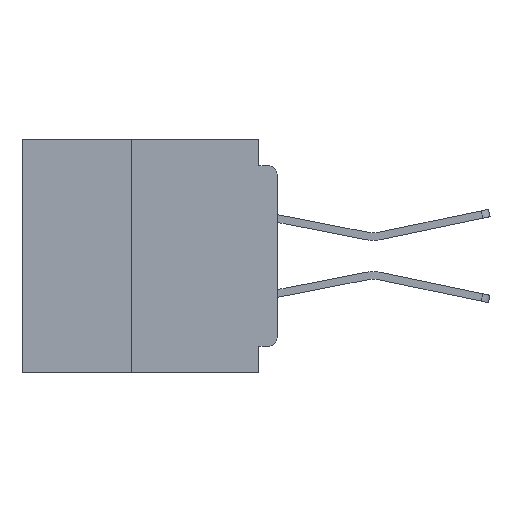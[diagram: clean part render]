
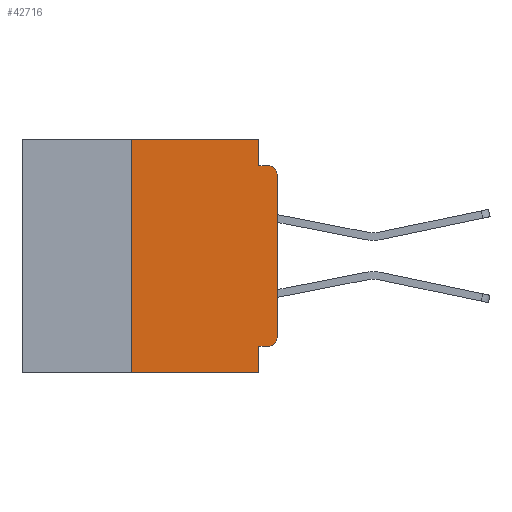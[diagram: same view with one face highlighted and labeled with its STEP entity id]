
A CAD part, left-side view. The second image highlights one B-rep face of the part: STEP entity #42716.
In plain terms, the highlighted planar face has unit normal (-1, 0, 0).
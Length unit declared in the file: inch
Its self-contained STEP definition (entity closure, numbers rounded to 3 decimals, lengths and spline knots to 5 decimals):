
#60 = CARTESIAN_POINT ( 'NONE',  ( 0., 0.015, -0.045 ) ) ;
#871 = ORIENTED_EDGE ( 'NONE', *, *, #28045, .T. ) ;
#939 = CARTESIAN_POINT ( 'NONE',  ( 0., 0., -0.355 ) ) ;
#1099 = CARTESIAN_POINT ( 'NONE',  ( 0., 0.031, -0.355 ) ) ;
#1116 = EDGE_CURVE ( 'NONE', #34935, #12988, #36839, .T. ) ;
#1674 = DIRECTION ( 'NONE',  ( 0., 1., 0. ) ) ;
#2947 = DIRECTION ( 'NONE',  ( 0., 0., 1. ) ) ;
#3328 = VERTEX_POINT ( 'NONE', #26756 ) ;
#4204 = CARTESIAN_POINT ( 'NONE',  ( 0., 0.031, 0. ) ) ;
#4971 = EDGE_LOOP ( 'NONE', ( #45256, #871, #13522, #13815, #39506, #6756, #7369, #54863, #20001, #50332 ) ) ;
#5549 = AXIS2_PLACEMENT_3D ( 'NONE', #36552, #10445, #40880 ) ;
#6756 = ORIENTED_EDGE ( 'NONE', *, *, #45501, .F. ) ;
#7180 = CARTESIAN_POINT ( 'NONE',  ( 0., 0.25, -0.4 ) ) ;
#7369 = ORIENTED_EDGE ( 'NONE', *, *, #21340, .T. ) ;
#7827 = CARTESIAN_POINT ( 'NONE',  ( 0., 0.031, 0. ) ) ;
#8248 = VERTEX_POINT ( 'NONE', #51144 ) ;
#9080 = VECTOR ( 'NONE', #18719, 39.37008 ) ;
#10445 = DIRECTION ( 'NONE',  ( -1., 0., 0. ) ) ;
#11455 = LINE ( 'NONE', #29660, #33284 ) ;
#12564 = CIRCLE ( 'NONE', #5549, 0.015 ) ;
#12753 = EDGE_CURVE ( 'NONE', #20427, #3328, #43786, .T. ) ;
#12988 = VERTEX_POINT ( 'NONE', #1099 ) ;
#13173 = LINE ( 'NONE', #17476, #23426 ) ;
#13522 = ORIENTED_EDGE ( 'NONE', *, *, #47722, .F. ) ;
#13557 = DIRECTION ( 'NONE',  ( 0., -1., 0. ) ) ;
#13815 = ORIENTED_EDGE ( 'NONE', *, *, #34812, .F. ) ;
#17476 = CARTESIAN_POINT ( 'NONE',  ( 0., 0.437, -0.4 ) ) ;
#18516 = EDGE_CURVE ( 'NONE', #36464, #53913, #11455, .T. ) ;
#18719 = DIRECTION ( 'NONE',  ( 0., 0., 1. ) ) ;
#18910 = AXIS2_PLACEMENT_3D ( 'NONE', #22741, #31313, #31490 ) ;
#20001 = ORIENTED_EDGE ( 'NONE', *, *, #1116, .F. ) ;
#20389 = VECTOR ( 'NONE', #49012, 39.37008 ) ;
#20427 = VERTEX_POINT ( 'NONE', #54319 ) ;
#21340 = EDGE_CURVE ( 'NONE', #31365, #35934, #13173, .T. ) ;
#21766 = LINE ( 'NONE', #31767, #20389 ) ;
#22258 = EDGE_CURVE ( 'NONE', #12988, #35934, #21766, .T. ) ;
#22369 = CARTESIAN_POINT ( 'NONE',  ( 0., 0., -0.045 ) ) ;
#22741 = CARTESIAN_POINT ( 'NONE',  ( 0., 0.437, 0. ) ) ;
#23426 = VECTOR ( 'NONE', #39134, 39.37008 ) ;
#24637 = VECTOR ( 'NONE', #2947, 39.37008 ) ;
#25216 = DIRECTION ( 'NONE',  ( 0., 0., -1. ) ) ;
#25240 = VECTOR ( 'NONE', #1674, 39.37008 ) ;
#25669 = CARTESIAN_POINT ( 'NONE',  ( 0., 0.015, -0.06 ) ) ;
#26756 = CARTESIAN_POINT ( 'NONE',  ( 0., 0., -0.06 ) ) ;
#27096 = PLANE ( 'NONE',  #18910 ) ;
#28045 = EDGE_CURVE ( 'NONE', #3328, #29928, #29028, .T. ) ;
#28723 = CARTESIAN_POINT ( 'NONE',  ( 0., 0.031, -0.4 ) ) ;
#29028 = CIRCLE ( 'NONE', #44156, 0.015 ) ;
#29503 = EDGE_CURVE ( 'NONE', #34935, #20427, #12564, .T. ) ;
#29660 = CARTESIAN_POINT ( 'NONE',  ( 0., 0.437, 0. ) ) ;
#29928 = VERTEX_POINT ( 'NONE', #60 ) ;
#30041 = DIRECTION ( 'NONE',  ( 0., 0., -1. ) ) ;
#31313 = DIRECTION ( 'NONE',  ( 1., 0., 0. ) ) ;
#31365 = VERTEX_POINT ( 'NONE', #36848 ) ;
#31490 = DIRECTION ( 'NONE',  ( 0., 0., -1. ) ) ;
#31625 = CARTESIAN_POINT ( 'NONE',  ( 0., 0., 0. ) ) ;
#31767 = CARTESIAN_POINT ( 'NONE',  ( 0., 0.031, -0.4 ) ) ;
#33284 = VECTOR ( 'NONE', #34023, 39.37008 ) ;
#34023 = DIRECTION ( 'NONE',  ( 0., -1., 0. ) ) ;
#34812 = EDGE_CURVE ( 'NONE', #53913, #8248, #37927, .T. ) ;
#34935 = VERTEX_POINT ( 'NONE', #52120 ) ;
#35934 = VERTEX_POINT ( 'NONE', #28723 ) ;
#36226 = LINE ( 'NONE', #7180, #24637 ) ;
#36368 = CARTESIAN_POINT ( 'NONE',  ( 0., 0.25, 0. ) ) ;
#36464 = VERTEX_POINT ( 'NONE', #36368 ) ;
#36552 = CARTESIAN_POINT ( 'NONE',  ( 0., 0.015, -0.34 ) ) ;
#36554 = VECTOR ( 'NONE', #25216, 39.37008 ) ;
#36839 = LINE ( 'NONE', #939, #25240 ) ;
#36848 = CARTESIAN_POINT ( 'NONE',  ( 0., 0.25, -0.4 ) ) ;
#37269 = FACE_OUTER_BOUND ( 'NONE', #4971, .T. ) ;
#37927 = LINE ( 'NONE', #7827, #36554 ) ;
#39134 = DIRECTION ( 'NONE',  ( 0., -1., 0. ) ) ;
#39506 = ORIENTED_EDGE ( 'NONE', *, *, #18516, .F. ) ;
#40880 = DIRECTION ( 'NONE',  ( 0., 0., -1. ) ) ;
#42716 = ADVANCED_FACE ( 'NONE', ( #37269 ), #27096, .F. ) ;
#43786 = LINE ( 'NONE', #31625, #9080 ) ;
#44156 = AXIS2_PLACEMENT_3D ( 'NONE', #25669, #55953, #30041 ) ;
#45256 = ORIENTED_EDGE ( 'NONE', *, *, #12753, .T. ) ;
#45501 = EDGE_CURVE ( 'NONE', #31365, #36464, #36226, .T. ) ;
#47722 = EDGE_CURVE ( 'NONE', #8248, #29928, #55636, .T. ) ;
#49012 = DIRECTION ( 'NONE',  ( 0., 0., -1. ) ) ;
#50332 = ORIENTED_EDGE ( 'NONE', *, *, #29503, .T. ) ;
#51144 = CARTESIAN_POINT ( 'NONE',  ( 0., 0.031, -0.045 ) ) ;
#52120 = CARTESIAN_POINT ( 'NONE',  ( 0., 0.015, -0.355 ) ) ;
#53913 = VERTEX_POINT ( 'NONE', #4204 ) ;
#54263 = VECTOR ( 'NONE', #13557, 39.37008 ) ;
#54319 = CARTESIAN_POINT ( 'NONE',  ( 0., 0., -0.34 ) ) ;
#54863 = ORIENTED_EDGE ( 'NONE', *, *, #22258, .F. ) ;
#55636 = LINE ( 'NONE', #22369, #54263 ) ;
#55953 = DIRECTION ( 'NONE',  ( -1., 0., 0. ) ) ;
